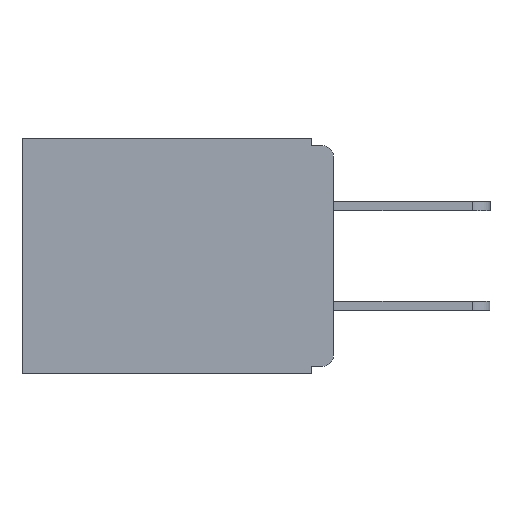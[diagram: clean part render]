
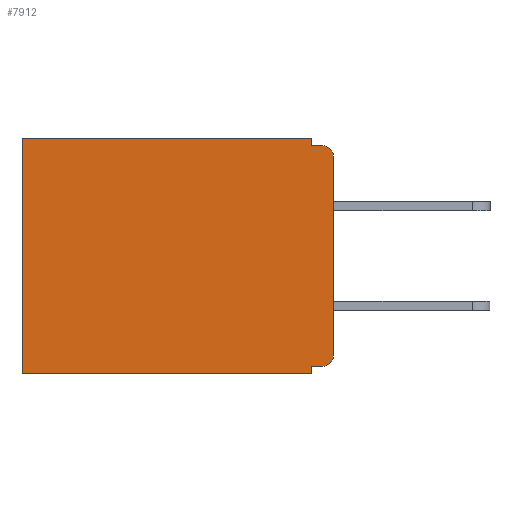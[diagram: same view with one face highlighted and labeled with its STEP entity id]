
A CAD part, left-side view. The second image highlights one B-rep face of the part: STEP entity #7912.
In plain terms, the highlighted planar face has unit normal (-1, 0, 0).
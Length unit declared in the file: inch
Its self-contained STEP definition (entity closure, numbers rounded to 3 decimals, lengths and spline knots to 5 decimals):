
#55 = CARTESIAN_POINT ( 'NONE',  ( 0.3, 0.031, 0. ) ) ;
#552 = ORIENTED_EDGE ( 'NONE', *, *, #4291, .F. ) ;
#675 = DIRECTION ( 'NONE',  ( 0., 0., -1. ) ) ;
#690 = ORIENTED_EDGE ( 'NONE', *, *, #1759, .F. ) ;
#831 = CARTESIAN_POINT ( 'NONE',  ( 0.3, 0., -0.32 ) ) ;
#887 = ORIENTED_EDGE ( 'NONE', *, *, #5167, .T. ) ;
#1188 = CARTESIAN_POINT ( 'NONE',  ( 0.3, 0.031, -0.01 ) ) ;
#1668 = VERTEX_POINT ( 'NONE', #10632 ) ;
#1671 = LINE ( 'NONE', #4397, #6639 ) ;
#1759 = EDGE_CURVE ( 'NONE', #7084, #8584, #11264, .T. ) ;
#1799 = CARTESIAN_POINT ( 'NONE',  ( 0.3, 0., -0.01 ) ) ;
#1974 = DIRECTION ( 'NONE',  ( 1., 0., 0. ) ) ;
#2124 = EDGE_CURVE ( 'NONE', #8584, #1668, #4845, .T. ) ;
#2411 = CARTESIAN_POINT ( 'NONE',  ( 0.3, 0.031, -0.33 ) ) ;
#2543 = EDGE_CURVE ( 'NONE', #3131, #10003, #10718, .T. ) ;
#2606 = VECTOR ( 'NONE', #12056, 39.37008 ) ;
#2921 = EDGE_CURVE ( 'NONE', #8895, #9327, #9011, .T. ) ;
#3014 = CARTESIAN_POINT ( 'NONE',  ( 0.3, 0.015, -0.305 ) ) ;
#3131 = VERTEX_POINT ( 'NONE', #9950 ) ;
#3716 = CIRCLE ( 'NONE', #8599, 0.015 ) ;
#4017 = DIRECTION ( 'NONE',  ( 0., 0., -1. ) ) ;
#4072 = ORIENTED_EDGE ( 'NONE', *, *, #2543, .F. ) ;
#4129 = VECTOR ( 'NONE', #9237, 39.37008 ) ;
#4153 = LINE ( 'NONE', #5304, #11427 ) ;
#4167 = EDGE_CURVE ( 'NONE', #5721, #12252, #10532, .T. ) ;
#4291 = EDGE_CURVE ( 'NONE', #8895, #6574, #1671, .T. ) ;
#4305 = CARTESIAN_POINT ( 'NONE',  ( 0.3, 0., 0. ) ) ;
#4397 = CARTESIAN_POINT ( 'NONE',  ( 0.3, 0., -0.33 ) ) ;
#4496 = ORIENTED_EDGE ( 'NONE', *, *, #6585, .F. ) ;
#4845 = LINE ( 'NONE', #2411, #7484 ) ;
#5151 = CARTESIAN_POINT ( 'NONE',  ( 0.3, 0.437, -0.33 ) ) ;
#5167 = EDGE_CURVE ( 'NONE', #7084, #6574, #3716, .T. ) ;
#5304 = CARTESIAN_POINT ( 'NONE',  ( 0.3, 0., -0.33 ) ) ;
#5357 = VECTOR ( 'NONE', #8755, 39.37008 ) ;
#5365 = DIRECTION ( 'NONE',  ( 0., 0., -1. ) ) ;
#5388 = EDGE_CURVE ( 'NONE', #1668, #12252, #4153, .T. ) ;
#5721 = VERTEX_POINT ( 'NONE', #9392 ) ;
#5806 = DIRECTION ( 'NONE',  ( 0., 1., 0. ) ) ;
#5987 = ORIENTED_EDGE ( 'NONE', *, *, #2921, .T. ) ;
#6122 = AXIS2_PLACEMENT_3D ( 'NONE', #7910, #1974, #8928 ) ;
#6262 = EDGE_CURVE ( 'NONE', #3131, #5721, #9088, .T. ) ;
#6574 = VERTEX_POINT ( 'NONE', #9714 ) ;
#6585 = EDGE_CURVE ( 'NONE', #10003, #9327, #7687, .T. ) ;
#6639 = VECTOR ( 'NONE', #5365, 39.37008 ) ;
#6642 = DIRECTION ( 'NONE',  ( -1., 0., 0. ) ) ;
#6824 = CARTESIAN_POINT ( 'NONE',  ( 0.3, 0., -0.025 ) ) ;
#7038 = DIRECTION ( 'NONE',  ( 0., 0., -1. ) ) ;
#7084 = VERTEX_POINT ( 'NONE', #8649 ) ;
#7189 = ORIENTED_EDGE ( 'NONE', *, *, #2124, .F. ) ;
#7368 = DIRECTION ( 'NONE',  ( 0., 0., -1. ) ) ;
#7484 = VECTOR ( 'NONE', #7368, 39.37008 ) ;
#7687 = LINE ( 'NONE', #1799, #5357 ) ;
#7910 = CARTESIAN_POINT ( 'NONE',  ( 0.3, 0., -0.33 ) ) ;
#7912 = ADVANCED_FACE ( 'NONE', ( #9680 ), #12823, .F. ) ;
#7994 = VECTOR ( 'NONE', #5806, 39.37008 ) ;
#8294 = DIRECTION ( 'NONE',  ( 0., 1., 0. ) ) ;
#8418 = VECTOR ( 'NONE', #7038, 39.37008 ) ;
#8447 = EDGE_LOOP ( 'NONE', ( #552, #5987, #4496, #4072, #11906, #10474, #10588, #7189, #690, #887 ) ) ;
#8580 = AXIS2_PLACEMENT_3D ( 'NONE', #12550, #6642, #675 ) ;
#8584 = VERTEX_POINT ( 'NONE', #9328 ) ;
#8599 = AXIS2_PLACEMENT_3D ( 'NONE', #3014, #9951, #4017 ) ;
#8649 = CARTESIAN_POINT ( 'NONE',  ( 0.3, 0.015, -0.32 ) ) ;
#8755 = DIRECTION ( 'NONE',  ( 0., -1., 0. ) ) ;
#8895 = VERTEX_POINT ( 'NONE', #6824 ) ;
#8928 = DIRECTION ( 'NONE',  ( 0., 0., -1. ) ) ;
#9011 = CIRCLE ( 'NONE', #8580, 0.015 ) ;
#9088 = LINE ( 'NONE', #4305, #4129 ) ;
#9237 = DIRECTION ( 'NONE',  ( 0., 1., 0. ) ) ;
#9327 = VERTEX_POINT ( 'NONE', #10512 ) ;
#9328 = CARTESIAN_POINT ( 'NONE',  ( 0.3, 0.031, -0.32 ) ) ;
#9392 = CARTESIAN_POINT ( 'NONE',  ( 0.3, 0.437, 0. ) ) ;
#9680 = FACE_OUTER_BOUND ( 'NONE', #8447, .T. ) ;
#9714 = CARTESIAN_POINT ( 'NONE',  ( 0.3, 0., -0.305 ) ) ;
#9950 = CARTESIAN_POINT ( 'NONE',  ( 0.3, 0.031, 0. ) ) ;
#9951 = DIRECTION ( 'NONE',  ( -1., 0., 0. ) ) ;
#10003 = VERTEX_POINT ( 'NONE', #1188 ) ;
#10474 = ORIENTED_EDGE ( 'NONE', *, *, #4167, .T. ) ;
#10512 = CARTESIAN_POINT ( 'NONE',  ( 0.3, 0.015, -0.01 ) ) ;
#10532 = LINE ( 'NONE', #5151, #2606 ) ;
#10588 = ORIENTED_EDGE ( 'NONE', *, *, #5388, .F. ) ;
#10632 = CARTESIAN_POINT ( 'NONE',  ( 0.3, 0.031, -0.33 ) ) ;
#10718 = LINE ( 'NONE', #55, #8418 ) ;
#11264 = LINE ( 'NONE', #831, #7994 ) ;
#11427 = VECTOR ( 'NONE', #8294, 39.37008 ) ;
#11710 = CARTESIAN_POINT ( 'NONE',  ( 0.3, 0.437, -0.33 ) ) ;
#11906 = ORIENTED_EDGE ( 'NONE', *, *, #6262, .T. ) ;
#12056 = DIRECTION ( 'NONE',  ( 0., 0., -1. ) ) ;
#12252 = VERTEX_POINT ( 'NONE', #11710 ) ;
#12550 = CARTESIAN_POINT ( 'NONE',  ( 0.3, 0.015, -0.025 ) ) ;
#12823 = PLANE ( 'NONE',  #6122 ) ;
